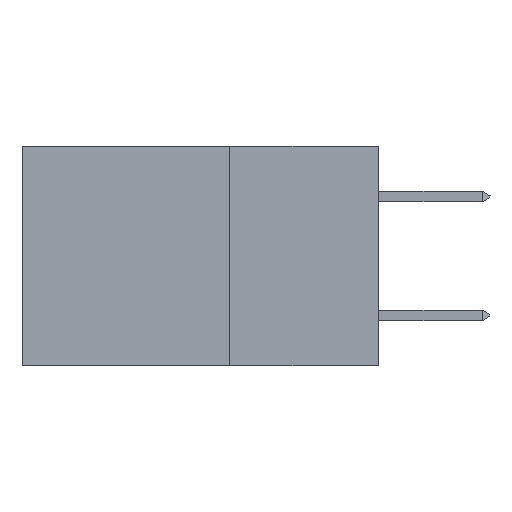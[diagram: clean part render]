
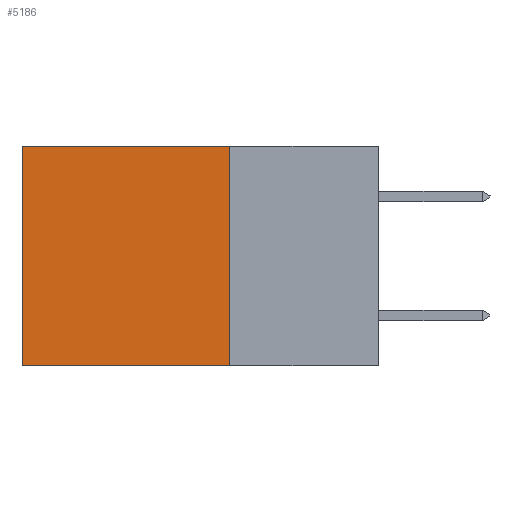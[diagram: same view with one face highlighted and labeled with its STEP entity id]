
A CAD part, left-side view. The second image highlights one B-rep face of the part: STEP entity #5186.
In plain terms, the highlighted planar face has unit normal (-1, 0, 0).
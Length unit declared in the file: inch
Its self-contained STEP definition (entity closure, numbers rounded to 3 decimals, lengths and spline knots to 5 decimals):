
#2 = FACE_OUTER_BOUND ( 'NONE', #483, .T. ) ;
#483 = EDGE_LOOP ( 'NONE', ( #8350, #14604, #12875, #4313 ) ) ;
#1269 = DIRECTION ( 'NONE',  ( 0., 0., -1. ) ) ;
#2233 = CARTESIAN_POINT ( 'NONE',  ( 0.2615, 0.6, 0. ) ) ;
#3284 = VECTOR ( 'NONE', #16029, 39.37008 ) ;
#3578 = VERTEX_POINT ( 'NONE', #16551 ) ;
#4313 = ORIENTED_EDGE ( 'NONE', *, *, #14396, .T. ) ;
#4435 = LINE ( 'NONE', #4549, #11649 ) ;
#4549 = CARTESIAN_POINT ( 'NONE',  ( 0.2615, 0.25, 0. ) ) ;
#5155 = AXIS2_PLACEMENT_3D ( 'NONE', #17358, #19126, #1269 ) ;
#5186 = ADVANCED_FACE ( 'NONE', ( #2 ), #19025, .F. ) ;
#5917 = CARTESIAN_POINT ( 'NONE',  ( 0.2615, 0.25, 0. ) ) ;
#5973 = DIRECTION ( 'NONE',  ( 0., 0., -1. ) ) ;
#6513 = LINE ( 'NONE', #6709, #3284 ) ;
#6622 = EDGE_CURVE ( 'NONE', #12480, #10637, #8995, .T. ) ;
#6709 = CARTESIAN_POINT ( 'NONE',  ( 0.2615, 0.25, -0.37 ) ) ;
#7153 = DIRECTION ( 'NONE',  ( 0., 0., -1. ) ) ;
#7975 = VECTOR ( 'NONE', #5973, 39.37008 ) ;
#8350 = ORIENTED_EDGE ( 'NONE', *, *, #18074, .T. ) ;
#8374 = VECTOR ( 'NONE', #7153, 39.37008 ) ;
#8894 = CARTESIAN_POINT ( 'NONE',  ( 0.2615, 0.25, -0.37 ) ) ;
#8995 = LINE ( 'NONE', #8894, #7975 ) ;
#10025 = EDGE_CURVE ( 'NONE', #10637, #3578, #6513, .T. ) ;
#10637 = VERTEX_POINT ( 'NONE', #20234 ) ;
#11649 = VECTOR ( 'NONE', #15853, 39.37008 ) ;
#11864 = LINE ( 'NONE', #15106, #8374 ) ;
#12480 = VERTEX_POINT ( 'NONE', #5917 ) ;
#12875 = ORIENTED_EDGE ( 'NONE', *, *, #6622, .F. ) ;
#14396 = EDGE_CURVE ( 'NONE', #12480, #19966, #4435, .T. ) ;
#14604 = ORIENTED_EDGE ( 'NONE', *, *, #10025, .F. ) ;
#15106 = CARTESIAN_POINT ( 'NONE',  ( 0.2615, 0.6, -0.37 ) ) ;
#15853 = DIRECTION ( 'NONE',  ( 0., 1., 0. ) ) ;
#16029 = DIRECTION ( 'NONE',  ( 0., 1., 0. ) ) ;
#16551 = CARTESIAN_POINT ( 'NONE',  ( 0.2615, 0.6, -0.37 ) ) ;
#17358 = CARTESIAN_POINT ( 'NONE',  ( 0.2615, 0.25, -0.37 ) ) ;
#18074 = EDGE_CURVE ( 'NONE', #19966, #3578, #11864, .T. ) ;
#19025 = PLANE ( 'NONE',  #5155 ) ;
#19126 = DIRECTION ( 'NONE',  ( 1., 0., 0. ) ) ;
#19966 = VERTEX_POINT ( 'NONE', #2233 ) ;
#20234 = CARTESIAN_POINT ( 'NONE',  ( 0.2615, 0.25, -0.37 ) ) ;
